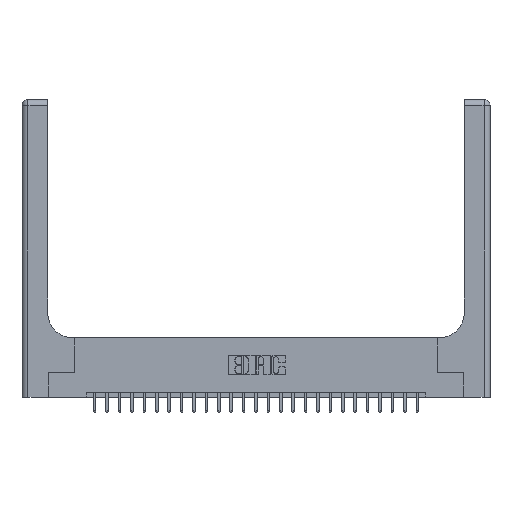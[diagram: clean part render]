
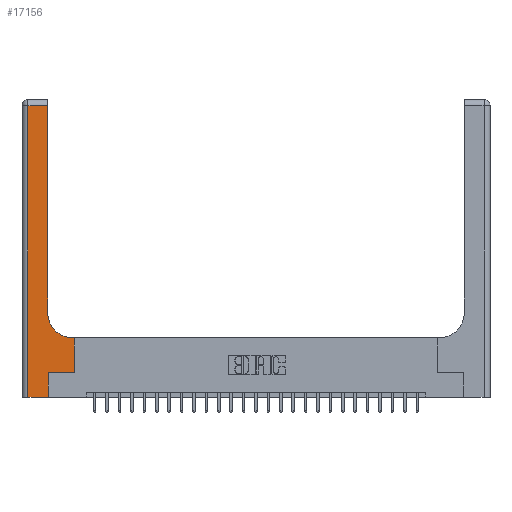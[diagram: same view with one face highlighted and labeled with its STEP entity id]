
A CAD part, top view. The second image highlights one B-rep face of the part: STEP entity #17156.
In plain terms, the highlighted planar face has unit normal (0, 0, 1).
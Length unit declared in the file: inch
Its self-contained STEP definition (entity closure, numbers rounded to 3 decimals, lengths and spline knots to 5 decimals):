
#340 = VERTEX_POINT ( 'NONE', #18898 ) ;
#852 = EDGE_CURVE ( 'NONE', #17813, #9497, #23307, .T. ) ;
#1076 = LINE ( 'NONE', #4383, #9206 ) ;
#1292 = CARTESIAN_POINT ( 'NONE',  ( 0., 3., 0.37 ) ) ;
#1308 = EDGE_CURVE ( 'NONE', #19338, #17813, #12456, .T. ) ;
#2145 = DIRECTION ( 'NONE',  ( 1., 0., 0. ) ) ;
#2374 = CARTESIAN_POINT ( 'NONE',  ( 0.51, 0.6, 0.37 ) ) ;
#3157 = EDGE_LOOP ( 'NONE', ( #22594, #19553, #22593, #20621, #20394, #13573, #24706, #3296, #4078 ) ) ;
#3211 = DIRECTION ( 'NONE',  ( -1., 0., 0. ) ) ;
#3296 = ORIENTED_EDGE ( 'NONE', *, *, #16594, .T. ) ;
#3308 = LINE ( 'NONE', #21264, #18041 ) ;
#3368 = AXIS2_PLACEMENT_3D ( 'NONE', #1292, #14712, #3211 ) ;
#3528 = CARTESIAN_POINT ( 'NONE',  ( 0.265, 0., 0.37 ) ) ;
#4004 = CARTESIAN_POINT ( 'NONE',  ( 0.06, 2.94, 0.37 ) ) ;
#4078 = ORIENTED_EDGE ( 'NONE', *, *, #23748, .T. ) ;
#4383 = CARTESIAN_POINT ( 'NONE',  ( 0., 2.94, 0.37 ) ) ;
#4792 = VERTEX_POINT ( 'NONE', #4004 ) ;
#4851 = CARTESIAN_POINT ( 'NONE',  ( 0.528, 0.25, 0.37 ) ) ;
#4875 = DIRECTION ( 'NONE',  ( 0., 1., 0. ) ) ;
#6402 = CARTESIAN_POINT ( 'NONE',  ( 0.528, 0.25, 0.37 ) ) ;
#7889 = VERTEX_POINT ( 'NONE', #2374 ) ;
#8252 = VERTEX_POINT ( 'NONE', #3528 ) ;
#8276 = EDGE_CURVE ( 'NONE', #8252, #19338, #3308, .T. ) ;
#8725 = CARTESIAN_POINT ( 'NONE',  ( 0.51, 0.85, 0.37 ) ) ;
#8906 = FACE_OUTER_BOUND ( 'NONE', #3157, .T. ) ;
#9206 = VECTOR ( 'NONE', #17668, 39.37008 ) ;
#9450 = CARTESIAN_POINT ( 'NONE',  ( 0.528, 0.6, 0.37 ) ) ;
#9497 = VERTEX_POINT ( 'NONE', #9450 ) ;
#9603 = DIRECTION ( 'NONE',  ( 0., 1., 0. ) ) ;
#9742 = CARTESIAN_POINT ( 'NONE',  ( 0.265, 0.25, 0.37 ) ) ;
#9946 = LINE ( 'NONE', #16106, #23414 ) ;
#10853 = PLANE ( 'NONE',  #3368 ) ;
#10996 = DIRECTION ( 'NONE',  ( 0., 0., -1. ) ) ;
#11290 = CARTESIAN_POINT ( 'NONE',  ( 0.26, 0.6, 0.37 ) ) ;
#11994 = EDGE_CURVE ( 'NONE', #20435, #340, #20278, .T. ) ;
#12456 = LINE ( 'NONE', #23196, #19107 ) ;
#12547 = VECTOR ( 'NONE', #19000, 39.37008 ) ;
#12662 = DIRECTION ( 'NONE',  ( 1., 0., 0. ) ) ;
#13223 = DIRECTION ( 'NONE',  ( -1., 0., 0. ) ) ;
#13359 = CARTESIAN_POINT ( 'NONE',  ( 0., 0., 0.37 ) ) ;
#13573 = ORIENTED_EDGE ( 'NONE', *, *, #1308, .T. ) ;
#13954 = VECTOR ( 'NONE', #4875, 39.37008 ) ;
#14065 = VERTEX_POINT ( 'NONE', #18575 ) ;
#14712 = DIRECTION ( 'NONE',  ( 0., 0., -1. ) ) ;
#15063 = EDGE_CURVE ( 'NONE', #4792, #14065, #9946, .T. ) ;
#16014 = AXIS2_PLACEMENT_3D ( 'NONE', #8725, #10996, #12662 ) ;
#16106 = CARTESIAN_POINT ( 'NONE',  ( 0.06, 3., 0.37 ) ) ;
#16495 = DIRECTION ( 'NONE',  ( 0., 1., 0. ) ) ;
#16594 = EDGE_CURVE ( 'NONE', #9497, #7889, #18246, .T. ) ;
#16728 = VECTOR ( 'NONE', #16495, 39.37008 ) ;
#17156 = ADVANCED_FACE ( 'NONE', ( #8906 ), #10853, .F. ) ;
#17402 = EDGE_CURVE ( 'NONE', #340, #4792, #1076, .T. ) ;
#17668 = DIRECTION ( 'NONE',  ( -1., 0., 0. ) ) ;
#17698 = LINE ( 'NONE', #13359, #12547 ) ;
#17813 = VERTEX_POINT ( 'NONE', #4851 ) ;
#18041 = VECTOR ( 'NONE', #9603, 39.37008 ) ;
#18098 = DIRECTION ( 'NONE',  ( 0., -1., 0. ) ) ;
#18246 = LINE ( 'NONE', #11290, #21265 ) ;
#18494 = CARTESIAN_POINT ( 'NONE',  ( 0.26, 3., 0.37 ) ) ;
#18575 = CARTESIAN_POINT ( 'NONE',  ( 0.06, 0., 0.37 ) ) ;
#18898 = CARTESIAN_POINT ( 'NONE',  ( 0.26, 2.94, 0.37 ) ) ;
#19000 = DIRECTION ( 'NONE',  ( 1., 0., 0. ) ) ;
#19107 = VECTOR ( 'NONE', #2145, 39.37008 ) ;
#19256 = CARTESIAN_POINT ( 'NONE',  ( 0.26, 0.85, 0.37 ) ) ;
#19338 = VERTEX_POINT ( 'NONE', #9742 ) ;
#19553 = ORIENTED_EDGE ( 'NONE', *, *, #17402, .T. ) ;
#20278 = LINE ( 'NONE', #18494, #13954 ) ;
#20394 = ORIENTED_EDGE ( 'NONE', *, *, #8276, .T. ) ;
#20435 = VERTEX_POINT ( 'NONE', #19256 ) ;
#20621 = ORIENTED_EDGE ( 'NONE', *, *, #21464, .T. ) ;
#21217 = CIRCLE ( 'NONE', #16014, 0.25 ) ;
#21264 = CARTESIAN_POINT ( 'NONE',  ( 0.265, 0., 0.37 ) ) ;
#21265 = VECTOR ( 'NONE', #13223, 39.37008 ) ;
#21464 = EDGE_CURVE ( 'NONE', #14065, #8252, #17698, .T. ) ;
#22593 = ORIENTED_EDGE ( 'NONE', *, *, #15063, .T. ) ;
#22594 = ORIENTED_EDGE ( 'NONE', *, *, #11994, .T. ) ;
#23196 = CARTESIAN_POINT ( 'NONE',  ( 0.265, 0.25, 0.37 ) ) ;
#23307 = LINE ( 'NONE', #6402, #16728 ) ;
#23414 = VECTOR ( 'NONE', #18098, 39.37008 ) ;
#23748 = EDGE_CURVE ( 'NONE', #7889, #20435, #21217, .T. ) ;
#24706 = ORIENTED_EDGE ( 'NONE', *, *, #852, .T. ) ;
